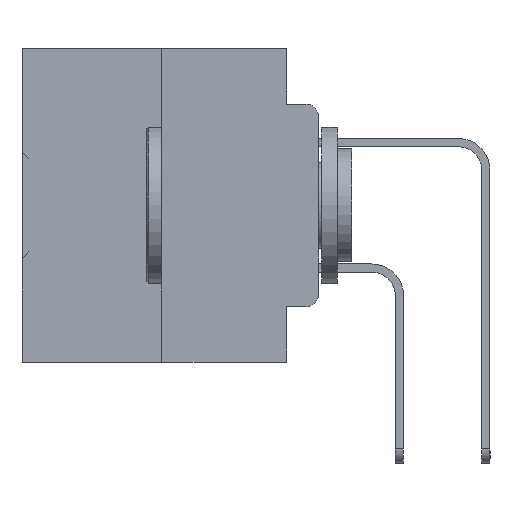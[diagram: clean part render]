
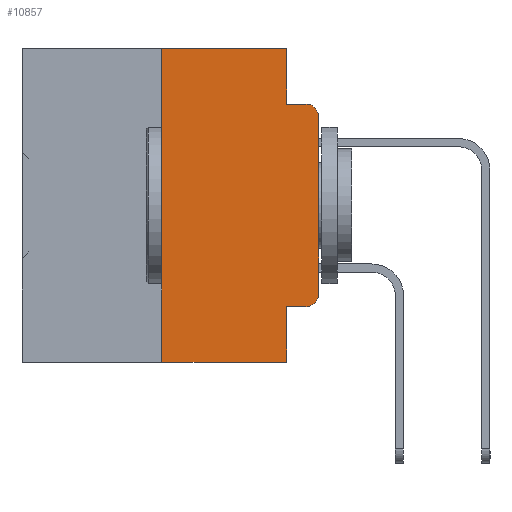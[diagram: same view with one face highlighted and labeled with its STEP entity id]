
A CAD part, left-side view. The second image highlights one B-rep face of the part: STEP entity #10857.
In plain terms, the highlighted planar face has unit normal (-1, 0, 0).
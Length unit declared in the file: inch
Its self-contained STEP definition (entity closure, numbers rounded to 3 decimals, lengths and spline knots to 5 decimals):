
#204 = VERTEX_POINT ( 'NONE', #22178 ) ;
#291 = CARTESIAN_POINT ( 'NONE',  ( 0., 0.473, 0. ) ) ;
#1470 = CARTESIAN_POINT ( 'NONE',  ( 0., 0.25, -0.5 ) ) ;
#1688 = CARTESIAN_POINT ( 'NONE',  ( 0., 0.051, 0. ) ) ;
#2106 = VECTOR ( 'NONE', #15039, 39.37008 ) ;
#2242 = CARTESIAN_POINT ( 'NONE',  ( 0., 0.02, -0.1085 ) ) ;
#2504 = CARTESIAN_POINT ( 'NONE',  ( 0., 0., -0.1085 ) ) ;
#2569 = CARTESIAN_POINT ( 'NONE',  ( 0., 0.473, 0. ) ) ;
#2718 = CARTESIAN_POINT ( 'NONE',  ( 0., 0.051, -0.0885 ) ) ;
#2763 = EDGE_CURVE ( 'NONE', #14419, #15318, #7004, .T. ) ;
#3784 = DIRECTION ( 'NONE',  ( 0., -1., 0. ) ) ;
#4138 = ORIENTED_EDGE ( 'NONE', *, *, #24628, .F. ) ;
#4382 = CARTESIAN_POINT ( 'NONE',  ( 0., 0.473, -0.5 ) ) ;
#4511 = EDGE_CURVE ( 'NONE', #14419, #38212, #26139, .T. ) ;
#5597 = FACE_OUTER_BOUND ( 'NONE', #11368, .T. ) ;
#5619 = ORIENTED_EDGE ( 'NONE', *, *, #39589, .T. ) ;
#6396 = CARTESIAN_POINT ( 'NONE',  ( 0., 0.051, -0.0885 ) ) ;
#6546 = VERTEX_POINT ( 'NONE', #6396 ) ;
#6768 = CARTESIAN_POINT ( 'NONE',  ( 0., 0.25, 0. ) ) ;
#7004 = LINE ( 'NONE', #4382, #19293 ) ;
#7101 = CIRCLE ( 'NONE', #22588, 0.02 ) ;
#7374 = VECTOR ( 'NONE', #36851, 39.37008 ) ;
#7407 = CARTESIAN_POINT ( 'NONE',  ( 0., 0., -0.3915 ) ) ;
#7413 = ORIENTED_EDGE ( 'NONE', *, *, #30979, .F. ) ;
#7770 = ORIENTED_EDGE ( 'NONE', *, *, #34067, .F. ) ;
#8994 = LINE ( 'NONE', #21922, #22501 ) ;
#9370 = VECTOR ( 'NONE', #26922, 39.37008 ) ;
#9585 = LINE ( 'NONE', #18658, #21889 ) ;
#10857 = ADVANCED_FACE ( 'NONE', ( #5597 ), #30256, .F. ) ;
#10919 = CARTESIAN_POINT ( 'NONE',  ( 0., 0.02, -0.4115 ) ) ;
#11368 = EDGE_LOOP ( 'NONE', ( #5619, #30005, #7413, #13808, #7770, #14123, #12302, #4138, #39788, #11456 ) ) ;
#11456 = ORIENTED_EDGE ( 'NONE', *, *, #32092, .T. ) ;
#11552 = DIRECTION ( 'NONE',  ( -1., 0., 0. ) ) ;
#12302 = ORIENTED_EDGE ( 'NONE', *, *, #2763, .T. ) ;
#13306 = DIRECTION ( 'NONE',  ( -1., 0., 0. ) ) ;
#13420 = CARTESIAN_POINT ( 'NONE',  ( 0., 0.051, -0.5 ) ) ;
#13808 = ORIENTED_EDGE ( 'NONE', *, *, #19372, .F. ) ;
#14123 = ORIENTED_EDGE ( 'NONE', *, *, #4511, .F. ) ;
#14419 = VERTEX_POINT ( 'NONE', #1470 ) ;
#14889 = DIRECTION ( 'NONE',  ( 1., 0., 0. ) ) ;
#15039 = DIRECTION ( 'NONE',  ( 0., -1., 0. ) ) ;
#15318 = VERTEX_POINT ( 'NONE', #13420 ) ;
#15456 = LINE ( 'NONE', #291, #7374 ) ;
#16877 = CARTESIAN_POINT ( 'NONE',  ( 0., 0.051, -0.4115 ) ) ;
#17817 = LINE ( 'NONE', #36391, #9370 ) ;
#18467 = DIRECTION ( 'NONE',  ( 0., 0., 1. ) ) ;
#18658 = CARTESIAN_POINT ( 'NONE',  ( 0., 0.051, 0. ) ) ;
#18882 = AXIS2_PLACEMENT_3D ( 'NONE', #28642, #13306, #37926 ) ;
#19011 = AXIS2_PLACEMENT_3D ( 'NONE', #2569, #14889, #28752 ) ;
#19073 = DIRECTION ( 'NONE',  ( 0., 0., 1. ) ) ;
#19293 = VECTOR ( 'NONE', #3784, 39.37008 ) ;
#19372 = EDGE_CURVE ( 'NONE', #34446, #6546, #17817, .T. ) ;
#20831 = DIRECTION ( 'NONE',  ( 0., 0., -1. ) ) ;
#21889 = VECTOR ( 'NONE', #31174, 39.37008 ) ;
#21922 = CARTESIAN_POINT ( 'NONE',  ( 0., 0., 0. ) ) ;
#22178 = CARTESIAN_POINT ( 'NONE',  ( 0., 0.051, -0.4115 ) ) ;
#22501 = VECTOR ( 'NONE', #18467, 39.37008 ) ;
#22588 = AXIS2_PLACEMENT_3D ( 'NONE', #2242, #11552, #20831 ) ;
#24573 = VERTEX_POINT ( 'NONE', #2504 ) ;
#24628 = EDGE_CURVE ( 'NONE', #204, #15318, #9585, .T. ) ;
#25722 = CARTESIAN_POINT ( 'NONE',  ( 0., 0.02, -0.0885 ) ) ;
#26139 = LINE ( 'NONE', #6768, #38241 ) ;
#26393 = LINE ( 'NONE', #16877, #32245 ) ;
#26895 = VERTEX_POINT ( 'NONE', #7407 ) ;
#26922 = DIRECTION ( 'NONE',  ( 0., 0., -1. ) ) ;
#27002 = EDGE_CURVE ( 'NONE', #204, #31612, #26393, .T. ) ;
#27453 = EDGE_CURVE ( 'NONE', #24573, #30284, #7101, .T. ) ;
#28642 = CARTESIAN_POINT ( 'NONE',  ( 0., 0.02, -0.3915 ) ) ;
#28752 = DIRECTION ( 'NONE',  ( 0., 0., -1. ) ) ;
#30005 = ORIENTED_EDGE ( 'NONE', *, *, #27453, .T. ) ;
#30256 = PLANE ( 'NONE',  #19011 ) ;
#30284 = VERTEX_POINT ( 'NONE', #25722 ) ;
#30484 = CIRCLE ( 'NONE', #18882, 0.02 ) ;
#30979 = EDGE_CURVE ( 'NONE', #6546, #30284, #33428, .T. ) ;
#31174 = DIRECTION ( 'NONE',  ( 0., 0., -1. ) ) ;
#31612 = VERTEX_POINT ( 'NONE', #10919 ) ;
#32092 = EDGE_CURVE ( 'NONE', #31612, #26895, #30484, .T. ) ;
#32245 = VECTOR ( 'NONE', #38696, 39.37008 ) ;
#33428 = LINE ( 'NONE', #2718, #2106 ) ;
#33609 = CARTESIAN_POINT ( 'NONE',  ( 0., 0.25, 0. ) ) ;
#34067 = EDGE_CURVE ( 'NONE', #38212, #34446, #15456, .T. ) ;
#34446 = VERTEX_POINT ( 'NONE', #1688 ) ;
#36391 = CARTESIAN_POINT ( 'NONE',  ( 0., 0.051, 0. ) ) ;
#36851 = DIRECTION ( 'NONE',  ( 0., -1., 0. ) ) ;
#37926 = DIRECTION ( 'NONE',  ( 0., 0., -1. ) ) ;
#38212 = VERTEX_POINT ( 'NONE', #33609 ) ;
#38241 = VECTOR ( 'NONE', #19073, 39.37008 ) ;
#38696 = DIRECTION ( 'NONE',  ( 0., -1., 0. ) ) ;
#39589 = EDGE_CURVE ( 'NONE', #26895, #24573, #8994, .T. ) ;
#39788 = ORIENTED_EDGE ( 'NONE', *, *, #27002, .T. ) ;
